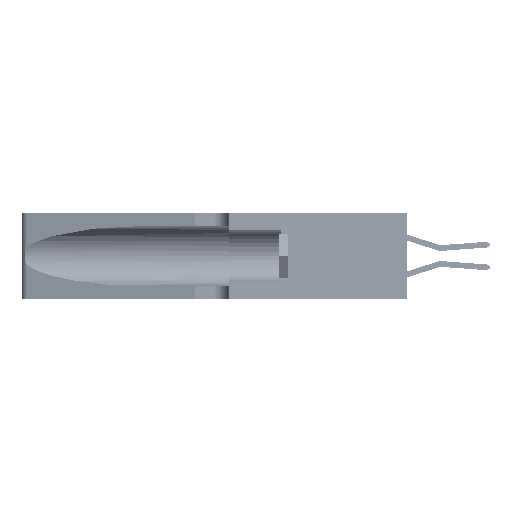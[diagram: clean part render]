
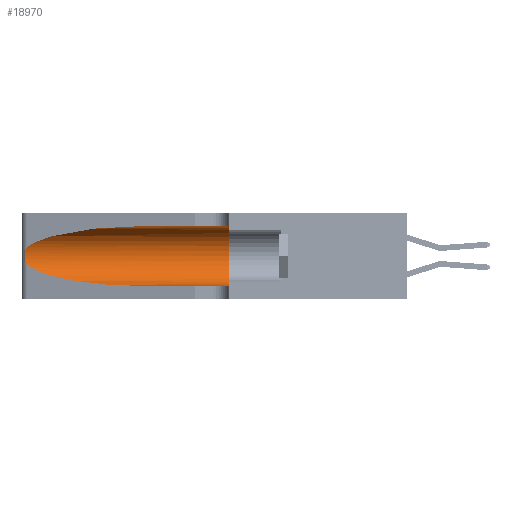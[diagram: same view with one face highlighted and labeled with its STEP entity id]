
A CAD part, left-side view. The second image highlights one B-rep face of the part: STEP entity #18970.
In plain terms, the highlighted cylindrical face has radius 3.308 mm (diameter 6.617 mm), a partial arc.
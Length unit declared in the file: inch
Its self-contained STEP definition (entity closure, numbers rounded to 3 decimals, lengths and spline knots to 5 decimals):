
#1387 = CARTESIAN_POINT ( 'NONE',  ( 0.18966, 0.96281, 0.31525 ) ) ;
#3749 = CARTESIAN_POINT ( 'NONE',  ( 0.25854, 1.2359, 0.20912 ) ) ;
#5831 = VECTOR ( 'NONE', #8565, 39.37008 ) ;
#6691 = VERTEX_POINT ( 'NONE', #17039 ) ;
#6979 = AXIS2_PLACEMENT_3D ( 'NONE', #19880, #53266, #44885 ) ;
#7983 = CARTESIAN_POINT ( 'NONE',  ( 0.26075, 1.23896, 0.19203 ) ) ;
#8473 = DIRECTION ( 'NONE',  ( 0., 1., 0. ) ) ;
#8565 = DIRECTION ( 'NONE',  ( 0., -1., 0. ) ) ;
#9182 = VERTEX_POINT ( 'NONE', #50742 ) ;
#10024 = CIRCLE ( 'NONE', #20483, 0.13025 ) ;
#11479 = EDGE_CURVE ( 'NONE', #15554, #21051, #51630, .T. ) ;
#12193 = CARTESIAN_POINT ( 'NONE',  ( 0.26017, 1.23833, 0.17102 ) ) ;
#14084 = CARTESIAN_POINT ( 'NONE',  ( 0.25487, 1.22718, 0.22369 ) ) ;
#14153 = CARTESIAN_POINT ( 'NONE',  ( 0.2373, 1.15595, 0.08982 ) ) ;
#15029 = B_SPLINE_CURVE_WITH_KNOTS ( 'NONE', 3,
 ( #20491, #24690, #53864, #28895, #3749, #33048, #7983, #37246, #12193, #41455, #16432, #45677, #20668, #49847 ),
 .UNSPECIFIED., .F., .F.,
 ( 4, 2, 2, 2, 2, 2, 4 ),
 ( 0., 0.00027, 0.00053, 0.00107, 0.0016, 0.00187, 0.00214 ),
 .UNSPECIFIED. ) ;
#15554 = VERTEX_POINT ( 'NONE', #16384 ) ;
#16266 = ORIENTED_EDGE ( 'NONE', *, *, #30431, .T. ) ;
#16384 = CARTESIAN_POINT ( 'NONE',  ( 0.1305, 0.72297, 0.05475 ) ) ;
#16432 = CARTESIAN_POINT ( 'NONE',  ( 0.25789, 1.23486, 0.15765 ) ) ;
#16602 = CARTESIAN_POINT ( 'NONE',  ( 0.1305, 0.35, 0.05475 ) ) ;
#17039 = CARTESIAN_POINT ( 'NONE',  ( 0.1305, 0.35, 0.31525 ) ) ;
#18970 = ADVANCED_FACE ( 'NONE', ( #23002 ), #35468, .F. ) ;
#19093 =( BOUNDED_CURVE ( )  B_SPLINE_CURVE ( 3, ( #51540, #1387, #39127, #14084 ),
 .UNSPECIFIED., .F., .T. ) 
 B_SPLINE_CURVE_WITH_KNOTS ( ( 4, 4 ),
 ( 1.5708, 2.84003 ),
 .UNSPECIFIED. ) 
 CURVE ( )  GEOMETRIC_REPRESENTATION_ITEM ( )  RATIONAL_B_SPLINE_CURVE ( ( 1., 0.87, 0.87, 1. ) ) 
 REPRESENTATION_ITEM ( '' )  );
#19880 = CARTESIAN_POINT ( 'NONE',  ( 0.1305, 1.61858, 0.185 ) ) ;
#20483 = AXIS2_PLACEMENT_3D ( 'NONE', #33541, #8473, #37746 ) ;
#20491 = CARTESIAN_POINT ( 'NONE',  ( 0.25487, 1.22718, 0.22369 ) ) ;
#20668 = CARTESIAN_POINT ( 'NONE',  ( 0.25555, 1.22993, 0.14849 ) ) ;
#21051 = VERTEX_POINT ( 'NONE', #16602 ) ;
#22601 = CARTESIAN_POINT ( 'NONE',  ( 0.1305, 0.72297, 0.05475 ) ) ;
#23002 = FACE_OUTER_BOUND ( 'NONE', #35057, .T. ) ;
#23031 = LINE ( 'NONE', #27021, #53675 ) ;
#23112 = ORIENTED_EDGE ( 'NONE', *, *, #11479, .T. ) ;
#24690 = CARTESIAN_POINT ( 'NONE',  ( 0.25555, 1.22994, 0.2215 ) ) ;
#25124 = DIRECTION ( 'NONE',  ( 0., -1., 0. ) ) ;
#27021 = CARTESIAN_POINT ( 'NONE',  ( 0.1305, 1.61858, 0.31525 ) ) ;
#27963 = EDGE_CURVE ( 'NONE', #43931, #15554, #38471, .T. ) ;
#28098 = ORIENTED_EDGE ( 'NONE', *, *, #31378, .F. ) ;
#28396 = EDGE_CURVE ( 'NONE', #43883, #6691, #23031, .T. ) ;
#28895 = CARTESIAN_POINT ( 'NONE',  ( 0.25787, 1.23484, 0.2124 ) ) ;
#30431 = EDGE_CURVE ( 'NONE', #43883, #9182, #19093, .T. ) ;
#31378 = EDGE_CURVE ( 'NONE', #6691, #21051, #10024, .T. ) ;
#33048 = CARTESIAN_POINT ( 'NONE',  ( 0.26018, 1.23835, 0.19895 ) ) ;
#33306 = ORIENTED_EDGE ( 'NONE', *, *, #27963, .T. ) ;
#33541 = CARTESIAN_POINT ( 'NONE',  ( 0.1305, 0.35, 0.185 ) ) ;
#34971 = CARTESIAN_POINT ( 'NONE',  ( 0.25487, 1.22718, 0.14631 ) ) ;
#35031 = CARTESIAN_POINT ( 'NONE',  ( 0.25487, 1.22718, 0.14631 ) ) ;
#35057 = EDGE_LOOP ( 'NONE', ( #16266, #51286, #33306, #23112, #28098, #38466 ) ) ;
#35468 = CYLINDRICAL_SURFACE ( 'NONE', #6979, 0.13025 ) ;
#37246 = CARTESIAN_POINT ( 'NONE',  ( 0.26075, 1.23896, 0.178 ) ) ;
#37746 = DIRECTION ( 'NONE',  ( 0., 0., 1. ) ) ;
#38466 = ORIENTED_EDGE ( 'NONE', *, *, #28396, .F. ) ;
#38471 =( BOUNDED_CURVE ( )  B_SPLINE_CURVE ( 3, ( #34971, #14153, #47596, #22601 ),
 .UNSPECIFIED., .F., .T. ) 
 B_SPLINE_CURVE_WITH_KNOTS ( ( 4, 4 ),
 ( 3.44316, 4.71239 ),
 .UNSPECIFIED. ) 
 CURVE ( )  GEOMETRIC_REPRESENTATION_ITEM ( )  RATIONAL_B_SPLINE_CURVE ( ( 1., 0.87, 0.87, 1. ) ) 
 REPRESENTATION_ITEM ( '' )  );
#39127 = CARTESIAN_POINT ( 'NONE',  ( 0.2373, 1.15595, 0.28018 ) ) ;
#41455 = CARTESIAN_POINT ( 'NONE',  ( 0.25856, 1.23593, 0.16098 ) ) ;
#43883 = VERTEX_POINT ( 'NONE', #51302 ) ;
#43931 = VERTEX_POINT ( 'NONE', #35031 ) ;
#44885 = DIRECTION ( 'NONE',  ( 0., 0., -1. ) ) ;
#45677 = CARTESIAN_POINT ( 'NONE',  ( 0.25639, 1.23186, 0.15144 ) ) ;
#46073 = CARTESIAN_POINT ( 'NONE',  ( 0.1305, 1.61858, 0.05475 ) ) ;
#47596 = CARTESIAN_POINT ( 'NONE',  ( 0.18966, 0.96281, 0.05475 ) ) ;
#48560 = EDGE_CURVE ( 'NONE', #9182, #43931, #15029, .T. ) ;
#49847 = CARTESIAN_POINT ( 'NONE',  ( 0.25487, 1.22718, 0.14631 ) ) ;
#50742 = CARTESIAN_POINT ( 'NONE',  ( 0.25487, 1.22718, 0.22369 ) ) ;
#51286 = ORIENTED_EDGE ( 'NONE', *, *, #48560, .T. ) ;
#51302 = CARTESIAN_POINT ( 'NONE',  ( 0.1305, 0.72297, 0.31525 ) ) ;
#51540 = CARTESIAN_POINT ( 'NONE',  ( 0.1305, 0.72297, 0.31525 ) ) ;
#51630 = LINE ( 'NONE', #46073, #5831 ) ;
#53266 = DIRECTION ( 'NONE',  ( 0., -1., 0. ) ) ;
#53675 = VECTOR ( 'NONE', #25124, 39.37008 ) ;
#53864 = CARTESIAN_POINT ( 'NONE',  ( 0.25639, 1.23184, 0.21858 ) ) ;
